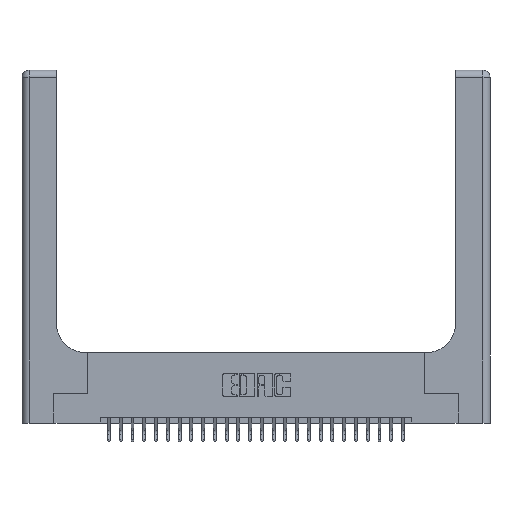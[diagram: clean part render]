
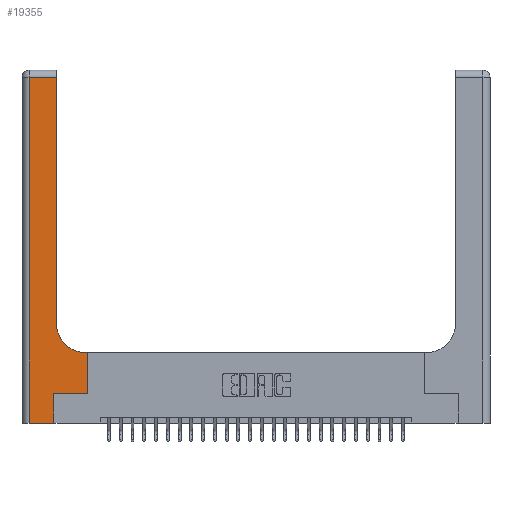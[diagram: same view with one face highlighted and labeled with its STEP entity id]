
A CAD part, top view. The second image highlights one B-rep face of the part: STEP entity #19355.
In plain terms, the highlighted planar face has unit normal (0, 0, 1).
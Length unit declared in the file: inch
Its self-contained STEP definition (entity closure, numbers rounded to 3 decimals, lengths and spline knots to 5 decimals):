
#12 = LINE ( 'NONE', #3432, #5165 ) ;
#89 = LINE ( 'NONE', #1008, #22419 ) ;
#108 = ORIENTED_EDGE ( 'NONE', *, *, #947, .T. ) ;
#582 = DIRECTION ( 'NONE',  ( 0., 1., 0. ) ) ;
#635 = VECTOR ( 'NONE', #582, 39.37008 ) ;
#679 = VECTOR ( 'NONE', #25375, 39.37008 ) ;
#947 = EDGE_CURVE ( 'NONE', #9917, #9616, #21638, .T. ) ;
#1008 = CARTESIAN_POINT ( 'NONE',  ( 0., 2.94, 0.37 ) ) ;
#1189 = VERTEX_POINT ( 'NONE', #11131 ) ;
#2303 = ORIENTED_EDGE ( 'NONE', *, *, #8570, .T. ) ;
#2538 = ORIENTED_EDGE ( 'NONE', *, *, #25757, .T. ) ;
#2607 = CARTESIAN_POINT ( 'NONE',  ( 0.5415, 0.85, 0.37 ) ) ;
#2855 = LINE ( 'NONE', #17101, #25788 ) ;
#3000 = CARTESIAN_POINT ( 'NONE',  ( 0.269, 0.25, 0.37 ) ) ;
#3151 = CIRCLE ( 'NONE', #14594, 0.25 ) ;
#3238 = PLANE ( 'NONE',  #14675 ) ;
#3432 = CARTESIAN_POINT ( 'NONE',  ( 0.06, 3., 0.37 ) ) ;
#3685 = EDGE_CURVE ( 'NONE', #1189, #9917, #24214, .T. ) ;
#3726 = DIRECTION ( 'NONE',  ( 0., 1., 0. ) ) ;
#4480 = VERTEX_POINT ( 'NONE', #6360 ) ;
#4806 = DIRECTION ( 'NONE',  ( 1., 0., 0. ) ) ;
#5165 = VECTOR ( 'NONE', #12059, 39.37008 ) ;
#5276 = ORIENTED_EDGE ( 'NONE', *, *, #26643, .T. ) ;
#5394 = CARTESIAN_POINT ( 'NONE',  ( 0.06, 2.94, 0.37 ) ) ;
#5454 = DIRECTION ( 'NONE',  ( 0., 0., -1. ) ) ;
#5831 = EDGE_CURVE ( 'NONE', #12374, #20888, #2855, .T. ) ;
#6020 = DIRECTION ( 'NONE',  ( 0., 1., 0. ) ) ;
#6157 = CARTESIAN_POINT ( 'NONE',  ( 0.5415, 0.6, 0.37 ) ) ;
#6360 = CARTESIAN_POINT ( 'NONE',  ( 0.2915, 2.94, 0.37 ) ) ;
#6973 = CARTESIAN_POINT ( 'NONE',  ( 0.269, 0., 0.37 ) ) ;
#7125 = LINE ( 'NONE', #11424, #635 ) ;
#7272 = ORIENTED_EDGE ( 'NONE', *, *, #21641, .T. ) ;
#8397 = VECTOR ( 'NONE', #3726, 39.37008 ) ;
#8417 = LINE ( 'NONE', #3000, #9788 ) ;
#8570 = EDGE_CURVE ( 'NONE', #24630, #4480, #7125, .T. ) ;
#9235 = CARTESIAN_POINT ( 'NONE',  ( 0.2915, 0.85, 0.37 ) ) ;
#9616 = VERTEX_POINT ( 'NONE', #6157 ) ;
#9788 = VECTOR ( 'NONE', #18115, 39.37008 ) ;
#9917 = VERTEX_POINT ( 'NONE', #24312 ) ;
#10646 = CARTESIAN_POINT ( 'NONE',  ( 0.269, 0.25, 0.37 ) ) ;
#11131 = CARTESIAN_POINT ( 'NONE',  ( 0.5585, 0.25, 0.37 ) ) ;
#11424 = CARTESIAN_POINT ( 'NONE',  ( 0.2915, 3., 0.37 ) ) ;
#12059 = DIRECTION ( 'NONE',  ( 0., -1., 0. ) ) ;
#12374 = VERTEX_POINT ( 'NONE', #21146 ) ;
#13522 = ORIENTED_EDGE ( 'NONE', *, *, #22298, .T. ) ;
#13639 = ORIENTED_EDGE ( 'NONE', *, *, #5831, .T. ) ;
#13994 = DIRECTION ( 'NONE',  ( -1., 0., 0. ) ) ;
#14462 = ORIENTED_EDGE ( 'NONE', *, *, #24320, .T. ) ;
#14594 = AXIS2_PLACEMENT_3D ( 'NONE', #2607, #17736, #4806 ) ;
#14675 = AXIS2_PLACEMENT_3D ( 'NONE', #20242, #5454, #20517 ) ;
#16673 = CARTESIAN_POINT ( 'NONE',  ( 0.5585, 0.25, 0.37 ) ) ;
#17101 = CARTESIAN_POINT ( 'NONE',  ( 0., 0., 0.37 ) ) ;
#17736 = DIRECTION ( 'NONE',  ( 0., 0., -1. ) ) ;
#18115 = DIRECTION ( 'NONE',  ( 1., 0., 0. ) ) ;
#18497 = EDGE_LOOP ( 'NONE', ( #2303, #7272, #5276, #13639, #14462, #13522, #23659, #108, #2538 ) ) ;
#18688 = VERTEX_POINT ( 'NONE', #5394 ) ;
#18982 = VERTEX_POINT ( 'NONE', #10646 ) ;
#19257 = DIRECTION ( 'NONE',  ( 1., 0., 0. ) ) ;
#19355 = ADVANCED_FACE ( 'NONE', ( #20547 ), #3238, .F. ) ;
#20242 = CARTESIAN_POINT ( 'NONE',  ( 0., 3., 0.37 ) ) ;
#20517 = DIRECTION ( 'NONE',  ( -1., 0., 0. ) ) ;
#20547 = FACE_OUTER_BOUND ( 'NONE', #18497, .T. ) ;
#20888 = VERTEX_POINT ( 'NONE', #6973 ) ;
#21085 = CARTESIAN_POINT ( 'NONE',  ( 0.269, 0., 0.37 ) ) ;
#21134 = VECTOR ( 'NONE', #6020, 39.37008 ) ;
#21146 = CARTESIAN_POINT ( 'NONE',  ( 0.06, 0., 0.37 ) ) ;
#21638 = LINE ( 'NONE', #25681, #679 ) ;
#21641 = EDGE_CURVE ( 'NONE', #4480, #18688, #89, .T. ) ;
#22298 = EDGE_CURVE ( 'NONE', #18982, #1189, #8417, .T. ) ;
#22419 = VECTOR ( 'NONE', #13994, 39.37008 ) ;
#23659 = ORIENTED_EDGE ( 'NONE', *, *, #3685, .T. ) ;
#24214 = LINE ( 'NONE', #16673, #8397 ) ;
#24312 = CARTESIAN_POINT ( 'NONE',  ( 0.5585, 0.6, 0.37 ) ) ;
#24320 = EDGE_CURVE ( 'NONE', #20888, #18982, #26854, .T. ) ;
#24630 = VERTEX_POINT ( 'NONE', #9235 ) ;
#25375 = DIRECTION ( 'NONE',  ( -1., 0., 0. ) ) ;
#25681 = CARTESIAN_POINT ( 'NONE',  ( 0.2915, 0.6, 0.37 ) ) ;
#25757 = EDGE_CURVE ( 'NONE', #9616, #24630, #3151, .T. ) ;
#25788 = VECTOR ( 'NONE', #19257, 39.37008 ) ;
#26643 = EDGE_CURVE ( 'NONE', #18688, #12374, #12, .T. ) ;
#26854 = LINE ( 'NONE', #21085, #21134 ) ;
